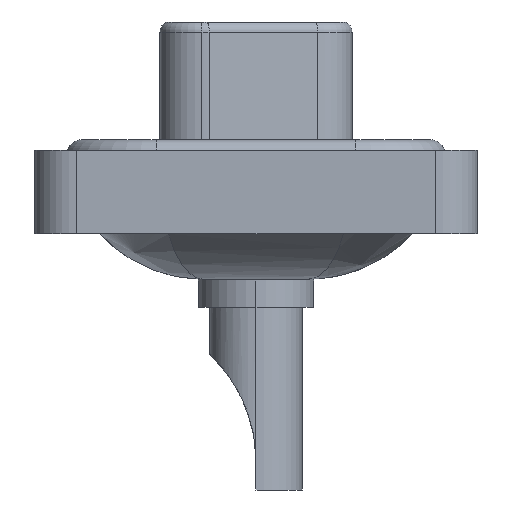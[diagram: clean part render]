
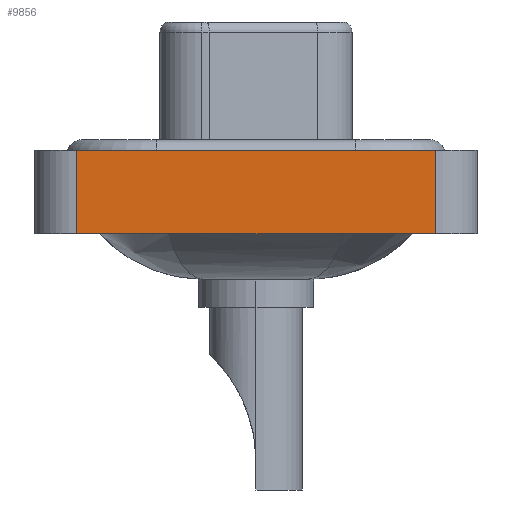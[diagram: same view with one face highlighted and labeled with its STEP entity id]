
A CAD part, left-side view. The second image highlights one B-rep face of the part: STEP entity #9856.
In plain terms, the highlighted planar face has unit normal (-1, 0, 0).
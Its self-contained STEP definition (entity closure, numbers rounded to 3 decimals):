
#42 = DIRECTION ( 'NONE',  ( 0., 0., 1. ) ) ;
#507 = EDGE_LOOP ( 'NONE', ( #11749, #5578, #3670, #12214 ) ) ;
#637 = DIRECTION ( 'NONE',  ( 0., -1., 0. ) ) ;
#1373 = EDGE_CURVE ( 'NONE', #6454, #16415, #2967, .T. ) ;
#2113 = CARTESIAN_POINT ( 'NONE',  ( -7.3, 8.55, -3.6 ) ) ;
#2267 = DIRECTION ( 'NONE',  ( -1., 0., 0. ) ) ;
#2429 = VECTOR ( 'NONE', #42, 1000. ) ;
#2967 = LINE ( 'NONE', #10388, #15186 ) ;
#3670 = ORIENTED_EDGE ( 'NONE', *, *, #7798, .F. ) ;
#3784 = EDGE_CURVE ( 'NONE', #16415, #13504, #17184, .T. ) ;
#3982 = CARTESIAN_POINT ( 'NONE',  ( -7.3, -8.55, 0.4 ) ) ;
#5260 = LINE ( 'NONE', #3982, #17990 ) ;
#5578 = ORIENTED_EDGE ( 'NONE', *, *, #15700, .F. ) ;
#6454 = VERTEX_POINT ( 'NONE', #2113 ) ;
#6740 = PLANE ( 'NONE',  #14057 ) ;
#7798 = EDGE_CURVE ( 'NONE', #6454, #17898, #13304, .T. ) ;
#9671 = DIRECTION ( 'NONE',  ( 0., 0., 1. ) ) ;
#9856 = ADVANCED_FACE ( 'NONE', ( #14340 ), #6740, .T. ) ;
#10028 = VECTOR ( 'NONE', #9671, 1000. ) ;
#10388 = CARTESIAN_POINT ( 'NONE',  ( -7.3, -8.55, -3.6 ) ) ;
#11749 = ORIENTED_EDGE ( 'NONE', *, *, #3784, .T. ) ;
#12214 = ORIENTED_EDGE ( 'NONE', *, *, #1373, .T. ) ;
#13304 = LINE ( 'NONE', #13685, #2429 ) ;
#13504 = VERTEX_POINT ( 'NONE', #15740 ) ;
#13685 = CARTESIAN_POINT ( 'NONE',  ( -7.3, 8.55, -3.6 ) ) ;
#14057 = AXIS2_PLACEMENT_3D ( 'NONE', #17301, #2267, #15828 ) ;
#14340 = FACE_OUTER_BOUND ( 'NONE', #507, .T. ) ;
#14942 = CARTESIAN_POINT ( 'NONE',  ( -7.3, 8.55, 0.4 ) ) ;
#15186 = VECTOR ( 'NONE', #16609, 1000. ) ;
#15700 = EDGE_CURVE ( 'NONE', #17898, #13504, #5260, .T. ) ;
#15740 = CARTESIAN_POINT ( 'NONE',  ( -7.3, -8.55, 0.4 ) ) ;
#15828 = DIRECTION ( 'NONE',  ( 0., 0., 1. ) ) ;
#15998 = CARTESIAN_POINT ( 'NONE',  ( -7.3, -8.55, -3.6 ) ) ;
#16415 = VERTEX_POINT ( 'NONE', #17504 ) ;
#16609 = DIRECTION ( 'NONE',  ( 0., -1., 0. ) ) ;
#17184 = LINE ( 'NONE', #15998, #10028 ) ;
#17301 = CARTESIAN_POINT ( 'NONE',  ( -7.3, -8.55, -3.6 ) ) ;
#17504 = CARTESIAN_POINT ( 'NONE',  ( -7.3, -8.55, -3.6 ) ) ;
#17898 = VERTEX_POINT ( 'NONE', #14942 ) ;
#17990 = VECTOR ( 'NONE', #637, 1000. ) ;
